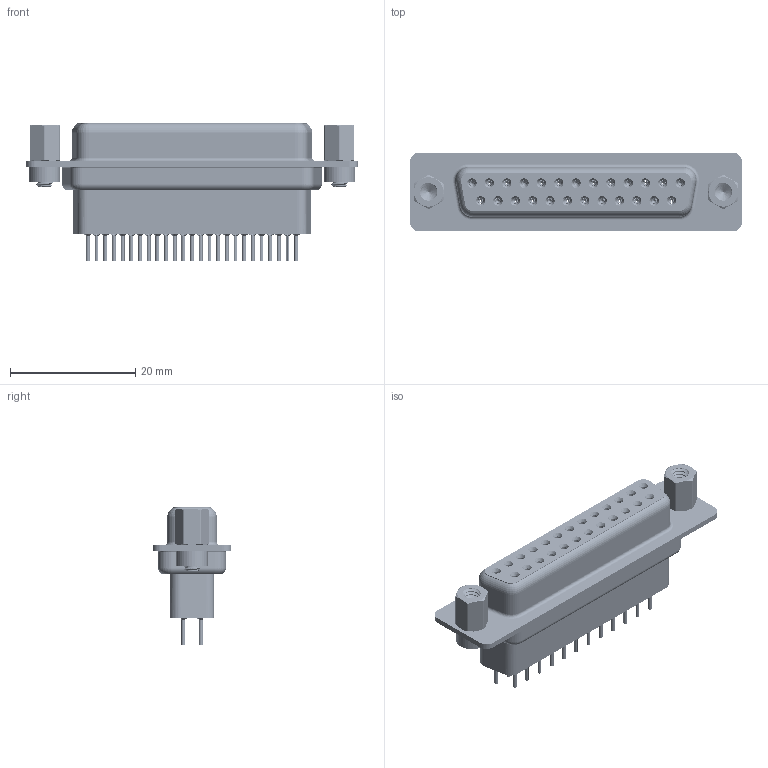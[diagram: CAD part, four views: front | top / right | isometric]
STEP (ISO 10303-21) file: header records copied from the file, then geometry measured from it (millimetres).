
FILE_DESCRIPTION (( 'STEP AP203' ), '1' );
FILE_NAME ('628-025-221-053.STEP', '2020-07-14T05:06:02', ( '' ), ( '' ), 'SwSTEP 2.0', 'SolidWorks 2020', '' );
FILE_SCHEMA (( 'CONFIG_CONTROL_DESIGN' ));
Length unit declared in the file: millimetre
Products named in the file (8): 628 Contact Row 1_21H; 628 Shell Front_25 Contacts; 628 Shell Rear_25 Contacts; 628 Housing_25 HP; 628 4-40 Threaded Rivet; 628 4-40 Hex Standoff; 628 Contact Row 2_21H; 628-025-221-053
Assembly tree (32 placements, depth 2):
  628-025-221-053
    628 Housing_25 HP
    628 Shell Front_25 Contacts
    628 Shell Rear_25 Contacts
    628 Contact Row 1_21H  x13
    628 Contact Row 2_21H  x12
    628 4-40 Threaded Rivet  x2
    628 4-40 Hex Standoff  x2
Bounding box: 53 x 12.6 x 21.9 mm (x, y, z)
Volume: 5193.3 mm3; surface area: 11954.4 mm2
Topology: 32 solids, 32 shells, 3476 faces, 8923 edges, 5572 vertices
Faces by surface type: cylinder 1032, plane 864, torus 657, bspline 518, cone 405
Entity records: 32569 total; most frequent: CARTESIAN_POINT 11119, DIRECTION 4327, ORIENTED_EDGE 4090, EDGE_CURVE 2045, AXIS2_PLACEMENT_3D 1804, VERTEX_POINT 1293, EDGE_LOOP 1002, CIRCLE 966
